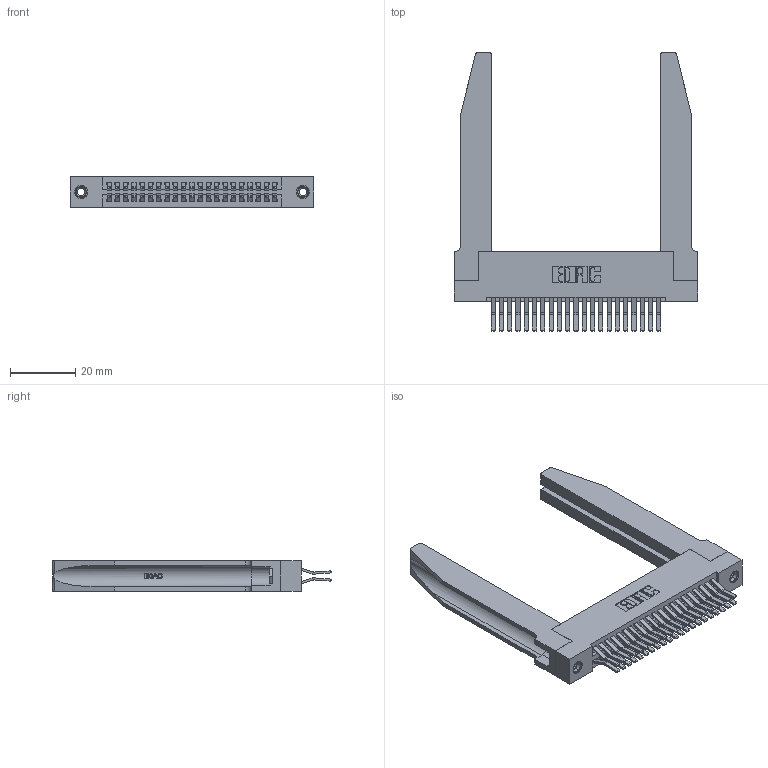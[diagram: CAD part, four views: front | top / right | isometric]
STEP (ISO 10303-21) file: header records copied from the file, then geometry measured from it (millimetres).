
FILE_DESCRIPTION (( 'STEP AP203' ), '1' );
FILE_NAME ('395-042-560-278.STEP', '2019-10-18T13:40:55', ( '' ), ( '' ), 'SwSTEP 2.0', 'SolidWorks 2016', '' );
FILE_SCHEMA (( 'CONFIG_CONTROL_DESIGN' ));
Length unit declared in the file: inch
Products named in the file (5): 345-220-078_345-220-078; 395-042-560-278; 345 Part_Flush Mounting Lugs - 0.156 Dia-TH; 345-292-001_560 Tail; 345-250-001_345-250-001-102
Assembly tree (47 placements, depth 2):
  395-042-560-278
    345 Part_Flush Mounting Lugs - 0.156 Dia-TH
    345-292-001_560 Tail  x42
    345-250-001_345-250-001-102  x2
    345-220-078_345-220-078  x2
Bounding box: 74.57 x 85.41 x 9.4 mm (x, y, z)
Volume: 15095 mm3; surface area: 17966.7 mm2
Topology: 47 solids, 47 shells, 2544 faces, 7459 edges, 4906 vertices
Faces by surface type: plane 1608, cylinder 884, bspline 36, cone 12, torus 4
Entity records: 24132 total; most frequent: CARTESIAN_POINT 4983, ORIENTED_EDGE 3814, DIRECTION 3417, EDGE_CURVE 1907, VECTOR 1593, LINE 1593, VERTEX_POINT 1264, AXIS2_PLACEMENT_3D 912
